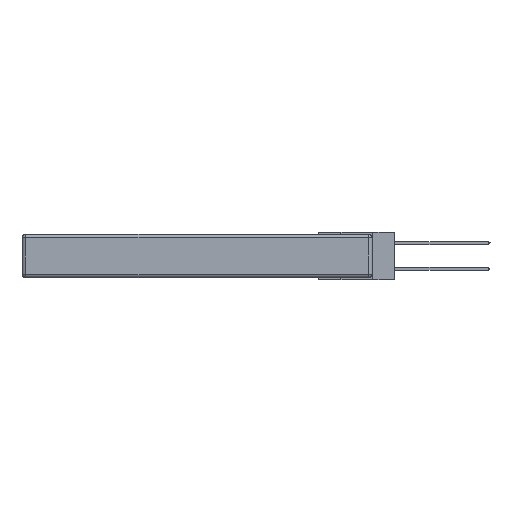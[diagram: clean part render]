
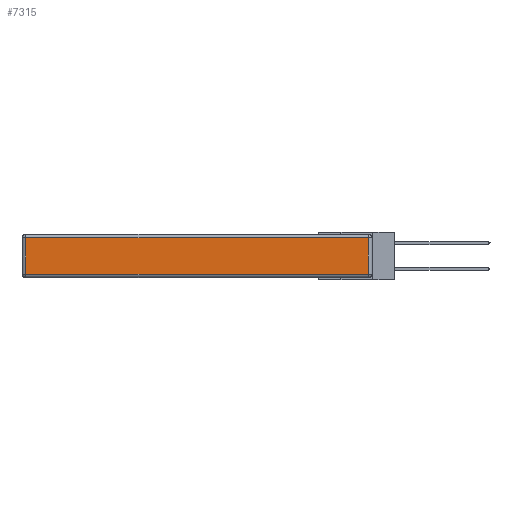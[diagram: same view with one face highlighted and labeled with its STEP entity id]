
A CAD part, left-side view. The second image highlights one B-rep face of the part: STEP entity #7315.
In plain terms, the highlighted planar face has unit normal (-1, 0, 0).
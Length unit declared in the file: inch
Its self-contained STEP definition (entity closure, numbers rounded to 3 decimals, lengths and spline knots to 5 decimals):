
#166 = EDGE_CURVE ( 'NONE', #1438, #6133, #11843, .T. ) ;
#249 = LINE ( 'NONE', #22060, #3387 ) ;
#518 = CARTESIAN_POINT ( 'NONE',  ( 0., 0.03, -0.313 ) ) ;
#906 = VECTOR ( 'NONE', #13811, 39.37008 ) ;
#1183 = ORIENTED_EDGE ( 'NONE', *, *, #22928, .T. ) ;
#1438 = VERTEX_POINT ( 'NONE', #19761 ) ;
#1948 = CARTESIAN_POINT ( 'NONE',  ( 0., 2.72, -0.03 ) ) ;
#2906 = CARTESIAN_POINT ( 'NONE',  ( 0., 0.03, -0.03 ) ) ;
#3387 = VECTOR ( 'NONE', #12695, 39.37008 ) ;
#3472 = VERTEX_POINT ( 'NONE', #1948 ) ;
#3492 = EDGE_CURVE ( 'NONE', #6133, #5556, #249, .T. ) ;
#3542 = ORIENTED_EDGE ( 'NONE', *, *, #13700, .T. ) ;
#4222 = CARTESIAN_POINT ( 'NONE',  ( 0., 2.75, -0.03 ) ) ;
#5556 = VERTEX_POINT ( 'NONE', #2906 ) ;
#5829 = ORIENTED_EDGE ( 'NONE', *, *, #166, .T. ) ;
#5858 = EDGE_LOOP ( 'NONE', ( #5829, #22728, #1183, #3542 ) ) ;
#6133 = VERTEX_POINT ( 'NONE', #518 ) ;
#6770 = VECTOR ( 'NONE', #9767, 39.37008 ) ;
#6922 = DIRECTION ( 'NONE',  ( 0., 0., 1. ) ) ;
#7315 = ADVANCED_FACE ( 'NONE', ( #12707 ), #14098, .T. ) ;
#9767 = DIRECTION ( 'NONE',  ( 0., 1., 0. ) ) ;
#10017 = CARTESIAN_POINT ( 'NONE',  ( 0., 2.72, -0.343 ) ) ;
#11263 = LINE ( 'NONE', #10017, #906 ) ;
#11843 = LINE ( 'NONE', #16037, #16219 ) ;
#12695 = DIRECTION ( 'NONE',  ( 0., 0., 1. ) ) ;
#12707 = FACE_OUTER_BOUND ( 'NONE', #5858, .T. ) ;
#13700 = EDGE_CURVE ( 'NONE', #3472, #1438, #11263, .T. ) ;
#13811 = DIRECTION ( 'NONE',  ( 0., 0., -1. ) ) ;
#14098 = PLANE ( 'NONE',  #19060 ) ;
#16037 = CARTESIAN_POINT ( 'NONE',  ( 0., 0., -0.313 ) ) ;
#16219 = VECTOR ( 'NONE', #19913, 39.37008 ) ;
#18607 = LINE ( 'NONE', #4222, #6770 ) ;
#19060 = AXIS2_PLACEMENT_3D ( 'NONE', #19769, #21564, #6922 ) ;
#19761 = CARTESIAN_POINT ( 'NONE',  ( 0., 2.72, -0.313 ) ) ;
#19769 = CARTESIAN_POINT ( 'NONE',  ( 0., 0., -0.343 ) ) ;
#19913 = DIRECTION ( 'NONE',  ( 0., -1., 0. ) ) ;
#21564 = DIRECTION ( 'NONE',  ( -1., 0., 0. ) ) ;
#22060 = CARTESIAN_POINT ( 'NONE',  ( 0., 0.03, -0.343 ) ) ;
#22728 = ORIENTED_EDGE ( 'NONE', *, *, #3492, .T. ) ;
#22928 = EDGE_CURVE ( 'NONE', #5556, #3472, #18607, .T. ) ;
